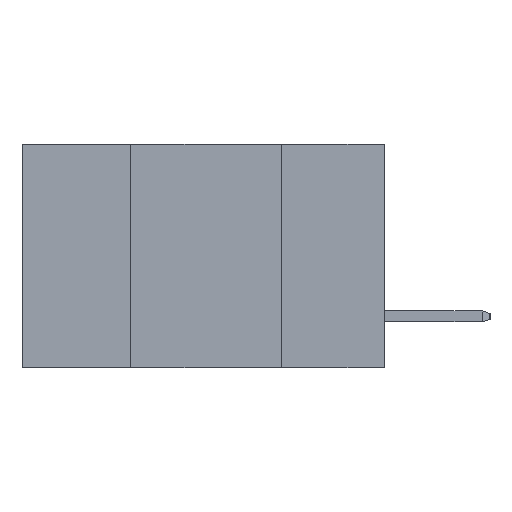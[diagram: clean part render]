
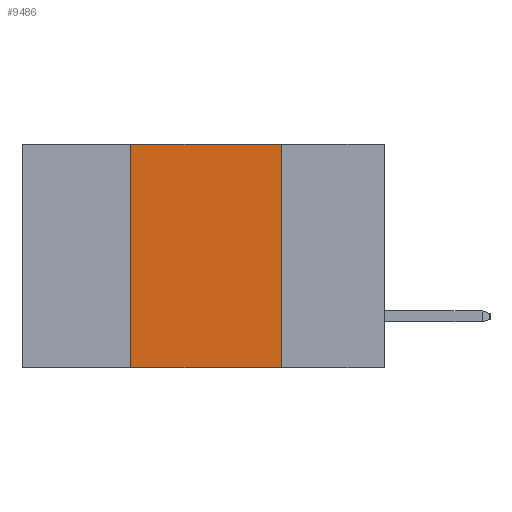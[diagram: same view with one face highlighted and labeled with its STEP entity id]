
A CAD part, left-side view. The second image highlights one B-rep face of the part: STEP entity #9486.
In plain terms, the highlighted planar face has unit normal (-1, 0, 0).
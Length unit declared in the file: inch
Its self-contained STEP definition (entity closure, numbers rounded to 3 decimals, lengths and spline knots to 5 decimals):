
#1448 = PLANE ( 'NONE',  #8693 ) ;
#1515 = LINE ( 'NONE', #3083, #10182 ) ;
#1729 = CARTESIAN_POINT ( 'NONE',  ( 0., 0.6, 0. ) ) ;
#1765 = EDGE_CURVE ( 'NONE', #12198, #12417, #6086, .T. ) ;
#2587 = CARTESIAN_POINT ( 'NONE',  ( 0., 0.6, 0. ) ) ;
#2771 = ORIENTED_EDGE ( 'NONE', *, *, #13713, .F. ) ;
#2834 = CARTESIAN_POINT ( 'NONE',  ( 0., 0.42, -0.37 ) ) ;
#2848 = DIRECTION ( 'NONE',  ( 0., -1., 0. ) ) ;
#3083 = CARTESIAN_POINT ( 'NONE',  ( 0., 0.17, -0.37 ) ) ;
#3099 = ORIENTED_EDGE ( 'NONE', *, *, #4489, .F. ) ;
#3537 = LINE ( 'NONE', #2834, #5112 ) ;
#3704 = DIRECTION ( 'NONE',  ( 0., 0., -1. ) ) ;
#4200 = DIRECTION ( 'NONE',  ( 0., 0., -1. ) ) ;
#4346 = ORIENTED_EDGE ( 'NONE', *, *, #6192, .F. ) ;
#4489 = EDGE_CURVE ( 'NONE', #12198, #13601, #3537, .T. ) ;
#5112 = VECTOR ( 'NONE', #6284, 39.37008 ) ;
#6086 = LINE ( 'NONE', #9616, #11759 ) ;
#6123 = LINE ( 'NONE', #1729, #11796 ) ;
#6192 = EDGE_CURVE ( 'NONE', #13601, #9905, #6123, .T. ) ;
#6284 = DIRECTION ( 'NONE',  ( 0., 0., 1. ) ) ;
#8208 = EDGE_LOOP ( 'NONE', ( #2771, #4346, #3099, #14034 ) ) ;
#8526 = CARTESIAN_POINT ( 'NONE',  ( 0., 0.17, -0.37 ) ) ;
#8693 = AXIS2_PLACEMENT_3D ( 'NONE', #2587, #10495, #3704 ) ;
#8932 = FACE_OUTER_BOUND ( 'NONE', #8208, .T. ) ;
#9163 = CARTESIAN_POINT ( 'NONE',  ( 0., 0.17, 0. ) ) ;
#9486 = ADVANCED_FACE ( 'NONE', ( #8932 ), #1448, .F. ) ;
#9533 = DIRECTION ( 'NONE',  ( 0., -1., 0. ) ) ;
#9616 = CARTESIAN_POINT ( 'NONE',  ( 0., 0.6, -0.37 ) ) ;
#9905 = VERTEX_POINT ( 'NONE', #9163 ) ;
#10182 = VECTOR ( 'NONE', #4200, 39.37008 ) ;
#10495 = DIRECTION ( 'NONE',  ( 1., 0., 0. ) ) ;
#11759 = VECTOR ( 'NONE', #9533, 39.37008 ) ;
#11796 = VECTOR ( 'NONE', #2848, 39.37008 ) ;
#11913 = CARTESIAN_POINT ( 'NONE',  ( 0., 0.42, 0. ) ) ;
#12198 = VERTEX_POINT ( 'NONE', #12555 ) ;
#12417 = VERTEX_POINT ( 'NONE', #8526 ) ;
#12555 = CARTESIAN_POINT ( 'NONE',  ( 0., 0.42, -0.37 ) ) ;
#13601 = VERTEX_POINT ( 'NONE', #11913 ) ;
#13713 = EDGE_CURVE ( 'NONE', #9905, #12417, #1515, .T. ) ;
#14034 = ORIENTED_EDGE ( 'NONE', *, *, #1765, .T. ) ;
